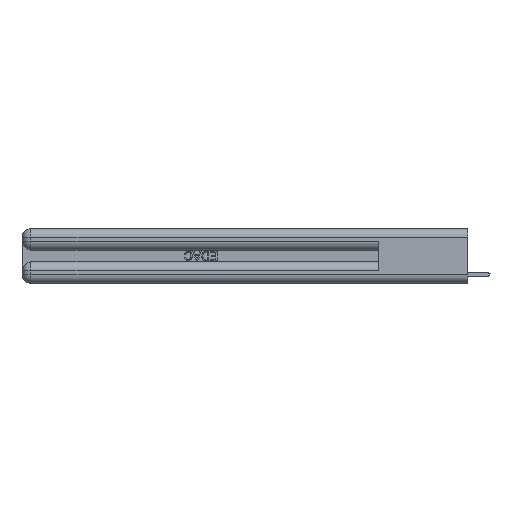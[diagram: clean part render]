
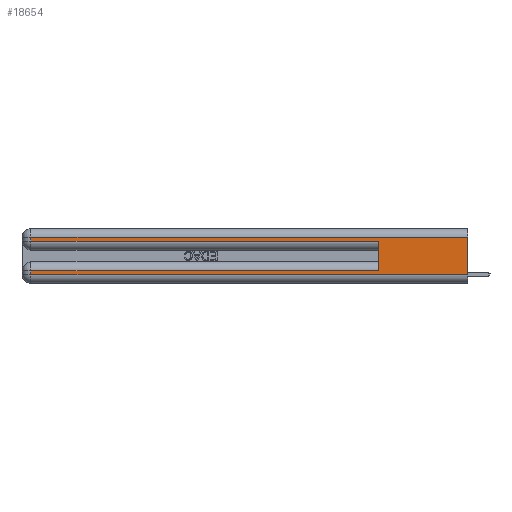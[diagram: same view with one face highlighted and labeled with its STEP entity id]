
A CAD part, left-side view. The second image highlights one B-rep face of the part: STEP entity #18654.
In plain terms, the highlighted planar face has unit normal (-1, 0, 0).
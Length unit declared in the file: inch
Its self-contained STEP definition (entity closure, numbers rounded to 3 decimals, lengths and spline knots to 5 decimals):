
#1126 = DIRECTION ( 'NONE',  ( 0., 0., -1. ) ) ;
#2220 = EDGE_CURVE ( 'NONE', #13367, #14682, #30805, .T. ) ;
#2302 = CARTESIAN_POINT ( 'NONE',  ( 0., 0.6, 0.285 ) ) ;
#2426 = VERTEX_POINT ( 'NONE', #21425 ) ;
#3483 = DIRECTION ( 'NONE',  ( 0., 0., -1. ) ) ;
#3616 = DIRECTION ( 'NONE',  ( 0., 1., 0. ) ) ;
#4184 = DIRECTION ( 'NONE',  ( 0., -1., 0. ) ) ;
#4189 = EDGE_CURVE ( 'NONE', #22498, #21026, #16656, .T. ) ;
#4605 = CARTESIAN_POINT ( 'NONE',  ( 0., 2.94, 0.31 ) ) ;
#5167 = EDGE_CURVE ( 'NONE', #13367, #2426, #25114, .T. ) ;
#5994 = CARTESIAN_POINT ( 'NONE',  ( 0., 0., 0.285 ) ) ;
#6077 = LINE ( 'NONE', #15101, #8303 ) ;
#6658 = VERTEX_POINT ( 'NONE', #26734 ) ;
#7095 = ORIENTED_EDGE ( 'NONE', *, *, #5167, .F. ) ;
#7231 = EDGE_CURVE ( 'NONE', #13584, #2426, #23792, .T. ) ;
#7926 = LINE ( 'NONE', #16246, #11315 ) ;
#8179 = CARTESIAN_POINT ( 'NONE',  ( 0., 0., 0.31 ) ) ;
#8303 = VECTOR ( 'NONE', #1126, 39.37008 ) ;
#8409 = ORIENTED_EDGE ( 'NONE', *, *, #2220, .T. ) ;
#10575 = DIRECTION ( 'NONE',  ( 0., 0., -1. ) ) ;
#11137 = LINE ( 'NONE', #27283, #29313 ) ;
#11240 = VECTOR ( 'NONE', #4184, 39.37008 ) ;
#11315 = VECTOR ( 'NONE', #30017, 39.37008 ) ;
#11522 = ORIENTED_EDGE ( 'NONE', *, *, #20559, .T. ) ;
#12440 = ORIENTED_EDGE ( 'NONE', *, *, #7231, .T. ) ;
#12556 = CARTESIAN_POINT ( 'NONE',  ( 0., 0., 0.31 ) ) ;
#12857 = CARTESIAN_POINT ( 'NONE',  ( 0., 0., 0.37 ) ) ;
#13367 = VERTEX_POINT ( 'NONE', #12556 ) ;
#13584 = VERTEX_POINT ( 'NONE', #15690 ) ;
#14037 = VECTOR ( 'NONE', #20456, 39.37008 ) ;
#14682 = VERTEX_POINT ( 'NONE', #4605 ) ;
#15101 = CARTESIAN_POINT ( 'NONE',  ( 0., 2.94, 0.37 ) ) ;
#15690 = CARTESIAN_POINT ( 'NONE',  ( 0., 2.94, 0.06 ) ) ;
#15943 = EDGE_CURVE ( 'NONE', #6658, #21026, #29365, .T. ) ;
#15973 = DIRECTION ( 'NONE',  ( 0., 0., -1. ) ) ;
#16246 = CARTESIAN_POINT ( 'NONE',  ( 0., 0., 0.085 ) ) ;
#16656 = LINE ( 'NONE', #5994, #14037 ) ;
#17113 = EDGE_CURVE ( 'NONE', #14682, #22498, #11137, .T. ) ;
#17456 = ORIENTED_EDGE ( 'NONE', *, *, #17113, .T. ) ;
#18271 = CARTESIAN_POINT ( 'NONE',  ( 0., 0., 0.37 ) ) ;
#18654 = ADVANCED_FACE ( 'NONE', ( #25849 ), #22597, .F. ) ;
#19417 = AXIS2_PLACEMENT_3D ( 'NONE', #12857, #29668, #3483 ) ;
#20440 = VECTOR ( 'NONE', #3616, 39.37008 ) ;
#20456 = DIRECTION ( 'NONE',  ( 0., -1., 0. ) ) ;
#20559 = EDGE_CURVE ( 'NONE', #28356, #13584, #6077, .T. ) ;
#21026 = VERTEX_POINT ( 'NONE', #2302 ) ;
#21425 = CARTESIAN_POINT ( 'NONE',  ( 0., 0., 0.06 ) ) ;
#21445 = ORIENTED_EDGE ( 'NONE', *, *, #4189, .T. ) ;
#22498 = VERTEX_POINT ( 'NONE', #25551 ) ;
#22597 = PLANE ( 'NONE',  #19417 ) ;
#22983 = CARTESIAN_POINT ( 'NONE',  ( 0., 0., 0.06 ) ) ;
#23792 = LINE ( 'NONE', #22983, #11240 ) ;
#24706 = VECTOR ( 'NONE', #15973, 39.37008 ) ;
#24900 = ORIENTED_EDGE ( 'NONE', *, *, #15943, .F. ) ;
#25114 = LINE ( 'NONE', #18271, #24706 ) ;
#25551 = CARTESIAN_POINT ( 'NONE',  ( 0., 2.94, 0.285 ) ) ;
#25849 = FACE_OUTER_BOUND ( 'NONE', #26507, .T. ) ;
#26447 = ORIENTED_EDGE ( 'NONE', *, *, #26650, .T. ) ;
#26507 = EDGE_LOOP ( 'NONE', ( #7095, #8409, #17456, #21445, #24900, #26447, #11522, #12440 ) ) ;
#26650 = EDGE_CURVE ( 'NONE', #6658, #28356, #7926, .T. ) ;
#26734 = CARTESIAN_POINT ( 'NONE',  ( 0., 0.6, 0.085 ) ) ;
#26760 = VECTOR ( 'NONE', #29549, 39.37008 ) ;
#27171 = CARTESIAN_POINT ( 'NONE',  ( 0., 0.6, 0.145 ) ) ;
#27283 = CARTESIAN_POINT ( 'NONE',  ( 0., 2.94, 0.37 ) ) ;
#28356 = VERTEX_POINT ( 'NONE', #29181 ) ;
#29181 = CARTESIAN_POINT ( 'NONE',  ( 0., 2.94, 0.085 ) ) ;
#29313 = VECTOR ( 'NONE', #10575, 39.37008 ) ;
#29365 = LINE ( 'NONE', #27171, #26760 ) ;
#29549 = DIRECTION ( 'NONE',  ( 0., 0., 1. ) ) ;
#29668 = DIRECTION ( 'NONE',  ( 1., 0., 0. ) ) ;
#30017 = DIRECTION ( 'NONE',  ( 0., 1., 0. ) ) ;
#30805 = LINE ( 'NONE', #8179, #20440 ) ;
